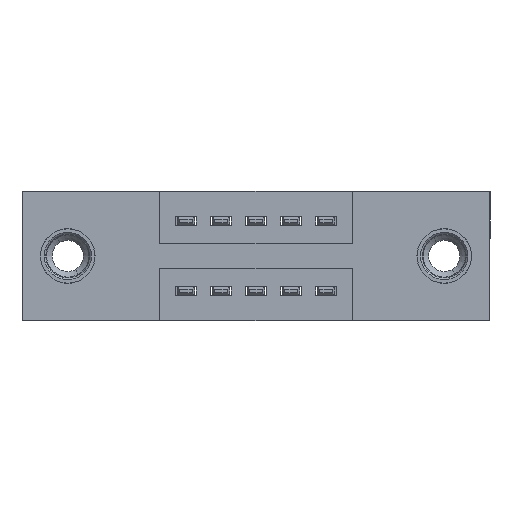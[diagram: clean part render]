
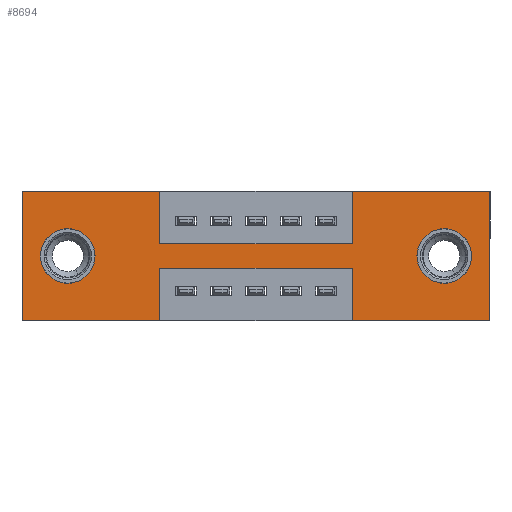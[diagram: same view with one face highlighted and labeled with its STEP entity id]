
A CAD part, front view. The second image highlights one B-rep face of the part: STEP entity #8694.
In plain terms, the highlighted planar face has unit normal (0, -1, 0).
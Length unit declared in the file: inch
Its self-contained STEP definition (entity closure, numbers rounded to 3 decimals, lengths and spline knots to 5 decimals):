
#26 = VERTEX_POINT ( 'NONE', #7194 ) ;
#44 = VECTOR ( 'NONE', #10602, 39.37008 ) ;
#115 = ORIENTED_EDGE ( 'NONE', *, *, #7839, .F. ) ;
#245 = VECTOR ( 'NONE', #9345, 39.37008 ) ;
#253 = CARTESIAN_POINT ( 'NONE',  ( 0.3925, 0., -0.15 ) ) ;
#312 = ORIENTED_EDGE ( 'NONE', *, *, #794, .F. ) ;
#324 = ORIENTED_EDGE ( 'NONE', *, *, #6540, .T. ) ;
#467 = CARTESIAN_POINT ( 'NONE',  ( 0.3925, 0., -0.22 ) ) ;
#513 = VERTEX_POINT ( 'NONE', #2780 ) ;
#530 = DIRECTION ( 'NONE',  ( 0., 0., 1. ) ) ;
#691 = CARTESIAN_POINT ( 'NONE',  ( 0.13, 0., -0.185 ) ) ;
#753 = DIRECTION ( 'NONE',  ( 1., 0., 0. ) ) ;
#785 = CARTESIAN_POINT ( 'NONE',  ( 1.335, 0., -0.37 ) ) ;
#794 = EDGE_CURVE ( 'NONE', #3805, #7169, #5063, .T. ) ;
#853 = EDGE_CURVE ( 'NONE', #6278, #7210, #2830, .T. ) ;
#965 = VECTOR ( 'NONE', #5723, 39.37008 ) ;
#1141 = DIRECTION ( 'NONE',  ( 1., 0., 0. ) ) ;
#1247 = VECTOR ( 'NONE', #7610, 39.37008 ) ;
#1271 = DIRECTION ( 'NONE',  ( 0., 0., -1. ) ) ;
#1398 = CARTESIAN_POINT ( 'NONE',  ( 1.335, 0., 0. ) ) ;
#1439 = CARTESIAN_POINT ( 'NONE',  ( 0.9425, 0., -0.37 ) ) ;
#1479 = LINE ( 'NONE', #253, #7932 ) ;
#1570 = ORIENTED_EDGE ( 'NONE', *, *, #8733, .F. ) ;
#1588 = DIRECTION ( 'NONE',  ( 0., 0., 1. ) ) ;
#1650 = CARTESIAN_POINT ( 'NONE',  ( 0.3925, 0., -0.37 ) ) ;
#1703 = DIRECTION ( 'NONE',  ( 0., 1., 0. ) ) ;
#2050 = VECTOR ( 'NONE', #10336, 39.37008 ) ;
#2099 = VERTEX_POINT ( 'NONE', #7663 ) ;
#2194 = CARTESIAN_POINT ( 'NONE',  ( 0.9425, 0., 0. ) ) ;
#2389 = LINE ( 'NONE', #4536, #8555 ) ;
#2467 = LINE ( 'NONE', #5586, #6921 ) ;
#2586 = CARTESIAN_POINT ( 'NONE',  ( 1.335, 0., 0. ) ) ;
#2647 = DIRECTION ( 'NONE',  ( 0., 1., 0. ) ) ;
#2725 = FACE_BOUND ( 'NONE', #4581, .T. ) ;
#2766 = ORIENTED_EDGE ( 'NONE', *, *, #3091, .T. ) ;
#2780 = CARTESIAN_POINT ( 'NONE',  ( 0., 0., 0. ) ) ;
#2799 = EDGE_LOOP ( 'NONE', ( #5948, #6929, #6100, #115, #9310, #5192, #8246, #2879, #312, #10324, #1570, #9407 ) ) ;
#2830 = LINE ( 'NONE', #8561, #245 ) ;
#2831 = CARTESIAN_POINT ( 'NONE',  ( 0., 0., -0.37 ) ) ;
#2879 = ORIENTED_EDGE ( 'NONE', *, *, #10431, .F. ) ;
#2893 = EDGE_CURVE ( 'NONE', #6697, #2099, #10106, .T. ) ;
#3040 = EDGE_CURVE ( 'NONE', #8229, #6294, #2389, .T. ) ;
#3081 = CARTESIAN_POINT ( 'NONE',  ( 0., 0., -0.37 ) ) ;
#3091 = EDGE_CURVE ( 'NONE', #10021, #6672, #9077, .T. ) ;
#3104 = VECTOR ( 'NONE', #1271, 39.37008 ) ;
#3266 = ORIENTED_EDGE ( 'NONE', *, *, #6607, .T. ) ;
#3283 = CARTESIAN_POINT ( 'NONE',  ( 1.205, 0., -0.107 ) ) ;
#3522 = FACE_OUTER_BOUND ( 'NONE', #2799, .T. ) ;
#3801 = CARTESIAN_POINT ( 'NONE',  ( 0.3925, 0., 0. ) ) ;
#3805 = VERTEX_POINT ( 'NONE', #3801 ) ;
#3809 = VERTEX_POINT ( 'NONE', #1398 ) ;
#3878 = EDGE_CURVE ( 'NONE', #2099, #6278, #9326, .T. ) ;
#3919 = DIRECTION ( 'NONE',  ( 0., -1., 0. ) ) ;
#4101 = DIRECTION ( 'NONE',  ( 0., 0., 1. ) ) ;
#4299 = LINE ( 'NONE', #2831, #2050 ) ;
#4536 = CARTESIAN_POINT ( 'NONE',  ( 0.9425, 0., 0. ) ) ;
#4575 = EDGE_CURVE ( 'NONE', #6294, #3809, #4600, .T. ) ;
#4581 = EDGE_LOOP ( 'NONE', ( #3266, #4634 ) ) ;
#4600 = LINE ( 'NONE', #6497, #44 ) ;
#4634 = ORIENTED_EDGE ( 'NONE', *, *, #4654, .T. ) ;
#4654 = EDGE_CURVE ( 'NONE', #26, #9958, #8284, .T. ) ;
#4849 = VERTEX_POINT ( 'NONE', #5197 ) ;
#4865 = VECTOR ( 'NONE', #9232, 39.37008 ) ;
#4928 = CARTESIAN_POINT ( 'NONE',  ( 0., 0., -0.37 ) ) ;
#5063 = LINE ( 'NONE', #8941, #3104 ) ;
#5192 = ORIENTED_EDGE ( 'NONE', *, *, #4575, .F. ) ;
#5197 = CARTESIAN_POINT ( 'NONE',  ( 0., 0., -0.37 ) ) ;
#5268 = CARTESIAN_POINT ( 'NONE',  ( 0.9425, 0., -0.37 ) ) ;
#5320 = EDGE_CURVE ( 'NONE', #513, #3805, #10821, .T. ) ;
#5458 = AXIS2_PLACEMENT_3D ( 'NONE', #6751, #1703, #7594 ) ;
#5586 = CARTESIAN_POINT ( 'NONE',  ( 0., 0., 0. ) ) ;
#5723 = DIRECTION ( 'NONE',  ( -1., 0., 0. ) ) ;
#5777 = DIRECTION ( 'NONE',  ( 0., 0., 1. ) ) ;
#5804 = AXIS2_PLACEMENT_3D ( 'NONE', #691, #6640, #1588 ) ;
#5839 = CARTESIAN_POINT ( 'NONE',  ( 0., 0., 0. ) ) ;
#5948 = ORIENTED_EDGE ( 'NONE', *, *, #853, .F. ) ;
#6100 = ORIENTED_EDGE ( 'NONE', *, *, #2893, .F. ) ;
#6278 = VERTEX_POINT ( 'NONE', #7237 ) ;
#6292 = AXIS2_PLACEMENT_3D ( 'NONE', #6745, #10533, #6509 ) ;
#6294 = VERTEX_POINT ( 'NONE', #2194 ) ;
#6387 = CARTESIAN_POINT ( 'NONE',  ( 0.13, 0., -0.107 ) ) ;
#6409 = LINE ( 'NONE', #2586, #1247 ) ;
#6430 = VECTOR ( 'NONE', #753, 39.37008 ) ;
#6497 = CARTESIAN_POINT ( 'NONE',  ( 0., 0., 0. ) ) ;
#6509 = DIRECTION ( 'NONE',  ( 0., 0., -1. ) ) ;
#6540 = EDGE_CURVE ( 'NONE', #6672, #10021, #10192, .T. ) ;
#6606 = AXIS2_PLACEMENT_3D ( 'NONE', #7672, #2647, #8502 ) ;
#6607 = EDGE_CURVE ( 'NONE', #9958, #26, #9691, .T. ) ;
#6640 = DIRECTION ( 'NONE',  ( 0., 1., 0. ) ) ;
#6672 = VERTEX_POINT ( 'NONE', #10221 ) ;
#6697 = VERTEX_POINT ( 'NONE', #5268 ) ;
#6745 = CARTESIAN_POINT ( 'NONE',  ( 1.205, 0., -0.185 ) ) ;
#6751 = CARTESIAN_POINT ( 'NONE',  ( 1.205, 0., -0.185 ) ) ;
#6921 = VECTOR ( 'NONE', #530, 39.37008 ) ;
#6929 = ORIENTED_EDGE ( 'NONE', *, *, #3878, .F. ) ;
#7169 = VERTEX_POINT ( 'NONE', #7511 ) ;
#7194 = CARTESIAN_POINT ( 'NONE',  ( 0.13, 0., -0.263 ) ) ;
#7210 = VERTEX_POINT ( 'NONE', #1650 ) ;
#7237 = CARTESIAN_POINT ( 'NONE',  ( 0.3925, 0., -0.22 ) ) ;
#7505 = EDGE_CURVE ( 'NONE', #7210, #4849, #9412, .T. ) ;
#7511 = CARTESIAN_POINT ( 'NONE',  ( 0.3925, 0., -0.15 ) ) ;
#7594 = DIRECTION ( 'NONE',  ( 0., 0., -1. ) ) ;
#7610 = DIRECTION ( 'NONE',  ( 0., 0., -1. ) ) ;
#7616 = EDGE_CURVE ( 'NONE', #3809, #9567, #6409, .T. ) ;
#7663 = CARTESIAN_POINT ( 'NONE',  ( 0.9425, 0., -0.22 ) ) ;
#7672 = CARTESIAN_POINT ( 'NONE',  ( 0.13, 0., -0.185 ) ) ;
#7839 = EDGE_CURVE ( 'NONE', #9567, #6697, #4299, .T. ) ;
#7908 = VECTOR ( 'NONE', #5777, 39.37008 ) ;
#7932 = VECTOR ( 'NONE', #1141, 39.37008 ) ;
#7951 = AXIS2_PLACEMENT_3D ( 'NONE', #3081, #3919, #9767 ) ;
#8109 = PLANE ( 'NONE',  #7951 ) ;
#8229 = VERTEX_POINT ( 'NONE', #10794 ) ;
#8246 = ORIENTED_EDGE ( 'NONE', *, *, #3040, .F. ) ;
#8284 = CIRCLE ( 'NONE', #5804, 0.078 ) ;
#8467 = EDGE_LOOP ( 'NONE', ( #2766, #324 ) ) ;
#8502 = DIRECTION ( 'NONE',  ( 0., 0., 1. ) ) ;
#8555 = VECTOR ( 'NONE', #4101, 39.37008 ) ;
#8561 = CARTESIAN_POINT ( 'NONE',  ( 0.3925, 0., -0.37 ) ) ;
#8694 = ADVANCED_FACE ( 'NONE', ( #9149, #2725, #3522 ), #8109, .T. ) ;
#8733 = EDGE_CURVE ( 'NONE', #4849, #513, #2467, .T. ) ;
#8941 = CARTESIAN_POINT ( 'NONE',  ( 0.3925, 0., 0. ) ) ;
#9077 = CIRCLE ( 'NONE', #6292, 0.078 ) ;
#9149 = FACE_BOUND ( 'NONE', #8467, .T. ) ;
#9232 = DIRECTION ( 'NONE',  ( -1., 0., 0. ) ) ;
#9310 = ORIENTED_EDGE ( 'NONE', *, *, #7616, .F. ) ;
#9326 = LINE ( 'NONE', #467, #4865 ) ;
#9345 = DIRECTION ( 'NONE',  ( 0., 0., -1. ) ) ;
#9407 = ORIENTED_EDGE ( 'NONE', *, *, #7505, .F. ) ;
#9412 = LINE ( 'NONE', #4928, #965 ) ;
#9567 = VERTEX_POINT ( 'NONE', #785 ) ;
#9691 = CIRCLE ( 'NONE', #6606, 0.078 ) ;
#9767 = DIRECTION ( 'NONE',  ( 0., 0., -1. ) ) ;
#9958 = VERTEX_POINT ( 'NONE', #6387 ) ;
#10021 = VERTEX_POINT ( 'NONE', #3283 ) ;
#10106 = LINE ( 'NONE', #1439, #7908 ) ;
#10192 = CIRCLE ( 'NONE', #5458, 0.078 ) ;
#10221 = CARTESIAN_POINT ( 'NONE',  ( 1.205, 0., -0.263 ) ) ;
#10324 = ORIENTED_EDGE ( 'NONE', *, *, #5320, .F. ) ;
#10336 = DIRECTION ( 'NONE',  ( -1., 0., 0. ) ) ;
#10431 = EDGE_CURVE ( 'NONE', #7169, #8229, #1479, .T. ) ;
#10533 = DIRECTION ( 'NONE',  ( 0., 1., 0. ) ) ;
#10602 = DIRECTION ( 'NONE',  ( 1., 0., 0. ) ) ;
#10794 = CARTESIAN_POINT ( 'NONE',  ( 0.9425, 0., -0.15 ) ) ;
#10821 = LINE ( 'NONE', #5839, #6430 ) ;
